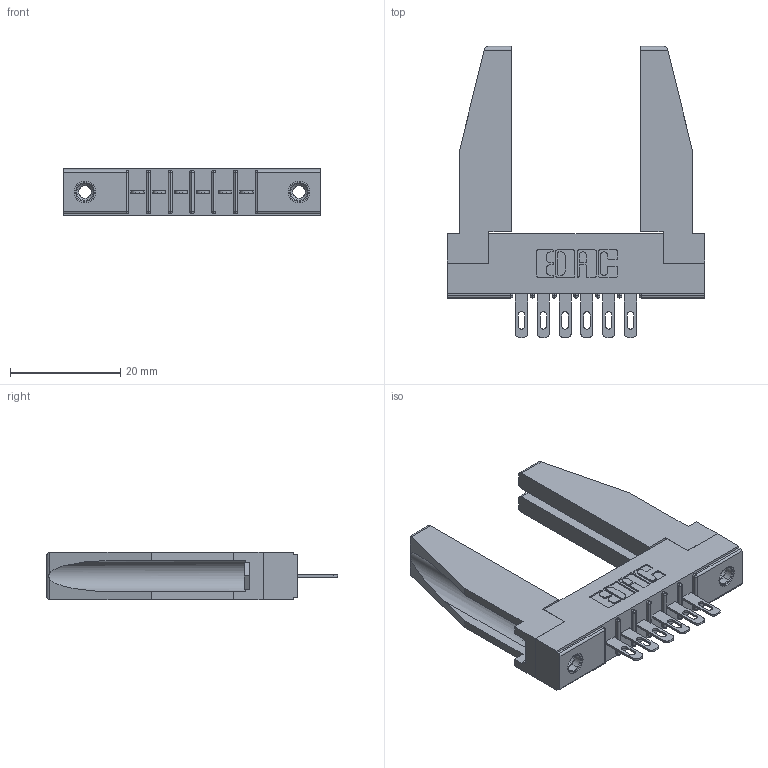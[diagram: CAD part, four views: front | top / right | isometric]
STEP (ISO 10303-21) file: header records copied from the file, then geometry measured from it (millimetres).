
FILE_DESCRIPTION (( 'STEP AP203' ), '1' );
FILE_NAME ('316-006-400-178.STEP', '2020-09-22T13:46:21', ( '' ), ( '' ), 'SwSTEP 2.0', 'SolidWorks 2020', '' );
FILE_SCHEMA (( 'CONFIG_CONTROL_DESIGN' ));
Length unit declared in the file: inch
Products named in the file (5): 345-250-001_345-250-001-102; 307-220-078; 316-006-400-178; 306-290-001_100; 306 Part_.156 Dia
Assembly tree (11 placements, depth 2):
  316-006-400-178
    306 Part_.156 Dia
    306-290-001_100  x6
    345-250-001_345-250-001-102  x2
    307-220-078  x2
Bounding box: 46.79 x 52.91 x 8.71 mm (x, y, z)
Volume: 7145.9 mm3; surface area: 8072.1 mm2
Topology: 11 solids, 11 shells, 702 faces, 1936 edges, 1248 vertices
Faces by surface type: plane 452, cylinder 210, sphere 24, cone 12, torus 4
Entity records: 12862 total; most frequent: CARTESIAN_POINT 2155, ORIENTED_EDGE 2090, DIRECTION 2081, EDGE_CURVE 1045, LINE 797, VECTOR 797, VERTEX_POINT 674, AXIS2_PLACEMENT_3D 642
